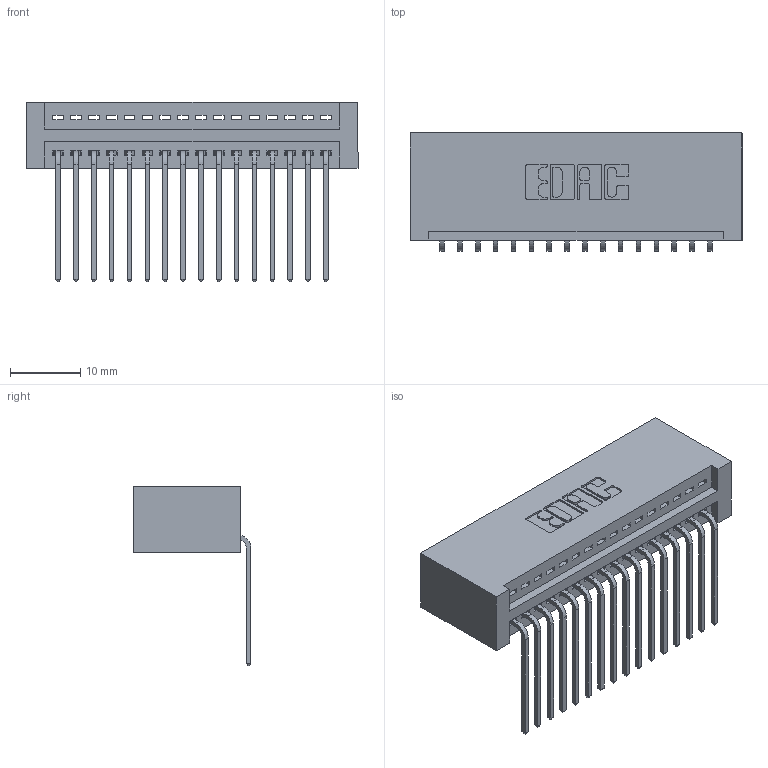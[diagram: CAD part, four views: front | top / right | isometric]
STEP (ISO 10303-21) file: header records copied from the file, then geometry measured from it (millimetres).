
FILE_DESCRIPTION (( 'STEP AP203' ), '1' );
FILE_NAME ('395-016-559-101.STEP', '2019-10-17T13:45:46', ( '' ), ( '' ), 'SwSTEP 2.0', 'SolidWorks 2016', '' );
FILE_SCHEMA (( 'CONFIG_CONTROL_DESIGN' ));
Length unit declared in the file: inch
Products named in the file (3): 345 Part_No Mounting Lugs; 345-292-001_558 559 Tail - 1; 395-016-559-101
Assembly tree (17 placements, depth 2):
  395-016-559-101
    345 Part_No Mounting Lugs
    345-292-001_558 559 Tail - 1  x16
Bounding box: 47.24 x 16.75 x 25.53 mm (x, y, z)
Volume: 4912 mm3; surface area: 6677.6 mm2
Topology: 17 solids, 17 shells, 1078 faces, 3229 edges, 2130 vertices
Faces by surface type: plane 748, cylinder 330
Entity records: 15349 total; most frequent: CARTESIAN_POINT 2668, ORIENTED_EDGE 2618, DIRECTION 2361, EDGE_CURVE 1309, LINE 1121, VECTOR 1121, VERTEX_POINT 870, AXIS2_PLACEMENT_3D 620
